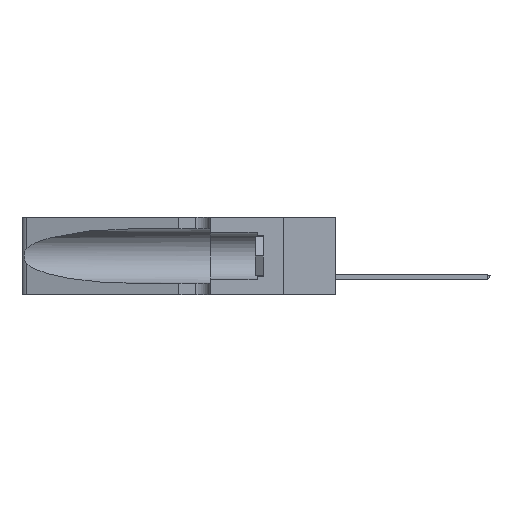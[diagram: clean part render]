
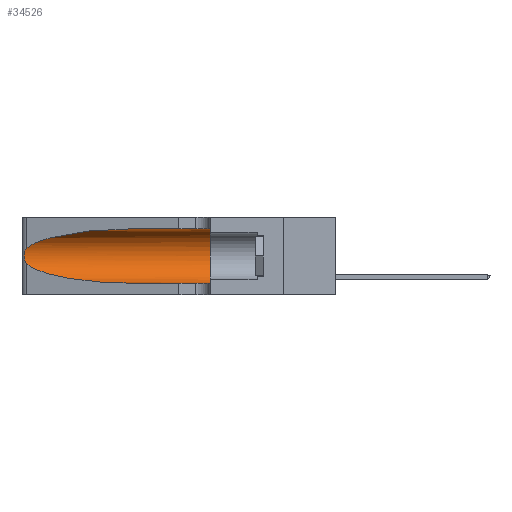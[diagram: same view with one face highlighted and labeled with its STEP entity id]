
A CAD part, left-side view. The second image highlights one B-rep face of the part: STEP entity #34526.
In plain terms, the highlighted cylindrical face has radius 3.308 mm (diameter 6.617 mm), a partial arc.
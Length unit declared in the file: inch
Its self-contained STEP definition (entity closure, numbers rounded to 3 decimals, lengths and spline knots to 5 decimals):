
#993 = CARTESIAN_POINT ( 'NONE',  ( 0.25487, 1.22718, 0.14631 ) ) ;
#2567 = VERTEX_POINT ( 'NONE', #50582 ) ;
#3283 = CARTESIAN_POINT ( 'NONE',  ( 0.2373, 1.15595, 0.28018 ) ) ;
#3933 = EDGE_CURVE ( 'NONE', #6805, #35640, #38484, .T. ) ;
#4226 = FACE_OUTER_BOUND ( 'NONE', #49511, .T. ) ;
#5020 = CARTESIAN_POINT ( 'NONE',  ( 0.1305, 0.72297, 0.05475 ) ) ;
#6805 = VERTEX_POINT ( 'NONE', #18992 ) ;
#7298 = CARTESIAN_POINT ( 'NONE',  ( 0.25487, 1.22718, 0.22369 ) ) ;
#7487 =( BOUNDED_CURVE ( )  B_SPLINE_CURVE ( 3, ( #40226, #11131, #3283, #7298 ),
 .UNSPECIFIED., .F., .F. ) 
 B_SPLINE_CURVE_WITH_KNOTS ( ( 4, 4 ),
 ( 1.5708, 2.84003 ),
 .UNSPECIFIED. ) 
 CURVE ( )  GEOMETRIC_REPRESENTATION_ITEM ( )  RATIONAL_B_SPLINE_CURVE ( ( 1., 0.87, 0.87, 1. ) ) 
 REPRESENTATION_ITEM ( '' )  );
#7595 = CARTESIAN_POINT ( 'NONE',  ( 0.26017, 1.23833, 0.17102 ) ) ;
#8194 = ORIENTED_EDGE ( 'NONE', *, *, #19451, .T. ) ;
#8409 = CARTESIAN_POINT ( 'NONE',  ( 0.25639, 1.23184, 0.21858 ) ) ;
#9734 = CARTESIAN_POINT ( 'NONE',  ( 0.25487, 1.22718, 0.14631 ) ) ;
#10050 = CARTESIAN_POINT ( 'NONE',  ( 0.26075, 1.23896, 0.19203 ) ) ;
#10239 = DIRECTION ( 'NONE',  ( 0., -1., 0. ) ) ;
#10698 = AXIS2_PLACEMENT_3D ( 'NONE', #34134, #42518, #19385 ) ;
#10859 = ORIENTED_EDGE ( 'NONE', *, *, #3933, .F. ) ;
#11131 = CARTESIAN_POINT ( 'NONE',  ( 0.18966, 0.96281, 0.31525 ) ) ;
#16436 = VERTEX_POINT ( 'NONE', #9734 ) ;
#18391 = VERTEX_POINT ( 'NONE', #46561 ) ;
#18992 = CARTESIAN_POINT ( 'NONE',  ( 0.1305, 0.35, 0.31525 ) ) ;
#19385 = DIRECTION ( 'NONE',  ( 0., 0., -1. ) ) ;
#19443 = CARTESIAN_POINT ( 'NONE',  ( 0.25639, 1.23186, 0.15144 ) ) ;
#19451 = EDGE_CURVE ( 'NONE', #2567, #35640, #44608, .T. ) ;
#24890 = CARTESIAN_POINT ( 'NONE',  ( 0.26018, 1.23835, 0.19895 ) ) ;
#25527 = CARTESIAN_POINT ( 'NONE',  ( 0.18966, 0.96281, 0.05475 ) ) ;
#26593 = ORIENTED_EDGE ( 'NONE', *, *, #36266, .T. ) ;
#26733 = CARTESIAN_POINT ( 'NONE',  ( 0.25856, 1.23593, 0.16098 ) ) ;
#28016 = EDGE_CURVE ( 'NONE', #49221, #18391, #7487, .T. ) ;
#28044 = ORIENTED_EDGE ( 'NONE', *, *, #28016, .T. ) ;
#28953 = EDGE_CURVE ( 'NONE', #49221, #6805, #39747, .T. ) ;
#29002 = CARTESIAN_POINT ( 'NONE',  ( 0.1305, 0.72297, 0.31525 ) ) ;
#29036 = CYLINDRICAL_SURFACE ( 'NONE', #10698, 0.13025 ) ;
#29148 = CARTESIAN_POINT ( 'NONE',  ( 0.2373, 1.15595, 0.08982 ) ) ;
#29229 = CARTESIAN_POINT ( 'NONE',  ( 0.1305, 0.35, 0.185 ) ) ;
#29761 = CARTESIAN_POINT ( 'NONE',  ( 0.25787, 1.23484, 0.2124 ) ) ;
#31286 = CARTESIAN_POINT ( 'NONE',  ( 0.25789, 1.23486, 0.15765 ) ) ;
#31625 = VECTOR ( 'NONE', #45774, 39.37008 ) ;
#33098 = DIRECTION ( 'NONE',  ( 0., 0., 1. ) ) ;
#33191 = CARTESIAN_POINT ( 'NONE',  ( 0.25555, 1.22994, 0.2215 ) ) ;
#33455 = DIRECTION ( 'NONE',  ( 0., 1., 0. ) ) ;
#34134 = CARTESIAN_POINT ( 'NONE',  ( 0.1305, 1.61858, 0.185 ) ) ;
#34526 = ADVANCED_FACE ( 'NONE', ( #4226 ), #29036, .F. ) ;
#35640 = VERTEX_POINT ( 'NONE', #48849 ) ;
#36266 = EDGE_CURVE ( 'NONE', #16436, #2567, #49840, .T. ) ;
#37216 = CARTESIAN_POINT ( 'NONE',  ( 0.1305, 1.61858, 0.05475 ) ) ;
#38484 = CIRCLE ( 'NONE', #47713, 0.13025 ) ;
#38612 = CARTESIAN_POINT ( 'NONE',  ( 0.25555, 1.22993, 0.14849 ) ) ;
#38982 = ORIENTED_EDGE ( 'NONE', *, *, #28953, .F. ) ;
#39747 = LINE ( 'NONE', #49530, #31625 ) ;
#40135 = CARTESIAN_POINT ( 'NONE',  ( 0.25854, 1.2359, 0.20912 ) ) ;
#40226 = CARTESIAN_POINT ( 'NONE',  ( 0.1305, 0.72297, 0.31525 ) ) ;
#42518 = DIRECTION ( 'NONE',  ( 0., -1., 0. ) ) ;
#42608 = CARTESIAN_POINT ( 'NONE',  ( 0.25487, 1.22718, 0.14631 ) ) ;
#43316 = CARTESIAN_POINT ( 'NONE',  ( 0.26075, 1.23896, 0.178 ) ) ;
#43988 = EDGE_CURVE ( 'NONE', #18391, #16436, #46077, .T. ) ;
#44608 = LINE ( 'NONE', #37216, #45198 ) ;
#45045 = ORIENTED_EDGE ( 'NONE', *, *, #43988, .T. ) ;
#45198 = VECTOR ( 'NONE', #10239, 39.37008 ) ;
#45774 = DIRECTION ( 'NONE',  ( 0., -1., 0. ) ) ;
#46077 = B_SPLINE_CURVE_WITH_KNOTS ( 'NONE', 3,
 ( #49013, #33191, #8409, #29761, #40135, #24890, #10050, #43316, #7595, #26733, #31286, #19443, #38612, #42608 ),
 .UNSPECIFIED., .F., .F.,
 ( 4, 2, 2, 2, 2, 2, 4 ),
 ( 0., 0.00027, 0.00053, 0.00107, 0.0016, 0.00187, 0.00214 ),
 .UNSPECIFIED. ) ;
#46561 = CARTESIAN_POINT ( 'NONE',  ( 0.25487, 1.22718, 0.22369 ) ) ;
#47713 = AXIS2_PLACEMENT_3D ( 'NONE', #29229, #33455, #33098 ) ;
#48849 = CARTESIAN_POINT ( 'NONE',  ( 0.1305, 0.35, 0.05475 ) ) ;
#49013 = CARTESIAN_POINT ( 'NONE',  ( 0.25487, 1.22718, 0.22369 ) ) ;
#49221 = VERTEX_POINT ( 'NONE', #29002 ) ;
#49511 = EDGE_LOOP ( 'NONE', ( #28044, #45045, #26593, #8194, #10859, #38982 ) ) ;
#49530 = CARTESIAN_POINT ( 'NONE',  ( 0.1305, 1.61858, 0.31525 ) ) ;
#49840 =( BOUNDED_CURVE ( )  B_SPLINE_CURVE ( 3, ( #993, #29148, #25527, #5020 ),
 .UNSPECIFIED., .F., .T. ) 
 B_SPLINE_CURVE_WITH_KNOTS ( ( 4, 4 ),
 ( 3.44316, 4.71239 ),
 .UNSPECIFIED. ) 
 CURVE ( )  GEOMETRIC_REPRESENTATION_ITEM ( )  RATIONAL_B_SPLINE_CURVE ( ( 1., 0.87, 0.87, 1. ) ) 
 REPRESENTATION_ITEM ( '' )  );
#50582 = CARTESIAN_POINT ( 'NONE',  ( 0.1305, 0.72297, 0.05475 ) ) ;
